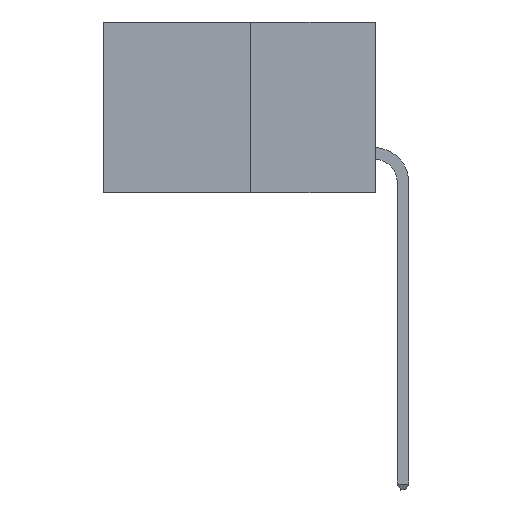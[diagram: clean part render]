
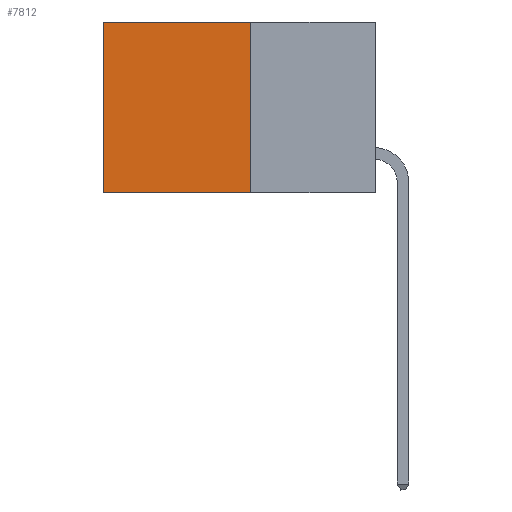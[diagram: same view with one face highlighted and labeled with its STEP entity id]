
A CAD part, left-side view. The second image highlights one B-rep face of the part: STEP entity #7812.
In plain terms, the highlighted planar face has unit normal (-1, 0, 0).
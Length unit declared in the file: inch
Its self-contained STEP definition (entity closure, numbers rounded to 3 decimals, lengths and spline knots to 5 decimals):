
#153 = VERTEX_POINT ( 'NONE', #9840 ) ;
#2208 = VECTOR ( 'NONE', #5039, 39.37008 ) ;
#2853 = EDGE_CURVE ( 'NONE', #7684, #153, #9256, .T. ) ;
#2869 = DIRECTION ( 'NONE',  ( 0., 0., -1. ) ) ;
#3282 = VECTOR ( 'NONE', #2869, 39.37008 ) ;
#3379 = CARTESIAN_POINT ( 'NONE',  ( 0.277, 0.27, -0.37 ) ) ;
#3427 = DIRECTION ( 'NONE',  ( 0., 0., -1. ) ) ;
#3918 = ORIENTED_EDGE ( 'NONE', *, *, #2853, .F. ) ;
#4128 = EDGE_LOOP ( 'NONE', ( #9489, #12944, #3918, #8191 ) ) ;
#5039 = DIRECTION ( 'NONE',  ( 0., 1., 0. ) ) ;
#5162 = DIRECTION ( 'NONE',  ( 0., 1., 0. ) ) ;
#5212 = CARTESIAN_POINT ( 'NONE',  ( 0.277, 0.59, 0. ) ) ;
#5635 = DIRECTION ( 'NONE',  ( 0., 0., -1. ) ) ;
#6323 = VERTEX_POINT ( 'NONE', #11208 ) ;
#6807 = VERTEX_POINT ( 'NONE', #5212 ) ;
#7485 = CARTESIAN_POINT ( 'NONE',  ( 0.277, 0.27, -0.37 ) ) ;
#7684 = VERTEX_POINT ( 'NONE', #11464 ) ;
#7806 = LINE ( 'NONE', #11505, #13668 ) ;
#7812 = ADVANCED_FACE ( 'NONE', ( #8192 ), #8173, .F. ) ;
#8173 = PLANE ( 'NONE',  #9640 ) ;
#8191 = ORIENTED_EDGE ( 'NONE', *, *, #9675, .T. ) ;
#8192 = FACE_OUTER_BOUND ( 'NONE', #4128, .T. ) ;
#9256 = LINE ( 'NONE', #3379, #3282 ) ;
#9312 = LINE ( 'NONE', #10989, #2208 ) ;
#9366 = CARTESIAN_POINT ( 'NONE',  ( 0.277, 0.27, -0.37 ) ) ;
#9489 = ORIENTED_EDGE ( 'NONE', *, *, #9718, .T. ) ;
#9640 = AXIS2_PLACEMENT_3D ( 'NONE', #9366, #10567, #3427 ) ;
#9675 = EDGE_CURVE ( 'NONE', #7684, #6807, #9312, .T. ) ;
#9718 = EDGE_CURVE ( 'NONE', #6807, #6323, #7806, .T. ) ;
#9840 = CARTESIAN_POINT ( 'NONE',  ( 0.277, 0.27, -0.37 ) ) ;
#10567 = DIRECTION ( 'NONE',  ( 1., 0., 0. ) ) ;
#10989 = CARTESIAN_POINT ( 'NONE',  ( 0.277, 0.27, 0. ) ) ;
#11208 = CARTESIAN_POINT ( 'NONE',  ( 0.277, 0.59, -0.37 ) ) ;
#11464 = CARTESIAN_POINT ( 'NONE',  ( 0.277, 0.27, 0. ) ) ;
#11505 = CARTESIAN_POINT ( 'NONE',  ( 0.277, 0.59, -0.37 ) ) ;
#11617 = EDGE_CURVE ( 'NONE', #153, #6323, #13819, .T. ) ;
#12944 = ORIENTED_EDGE ( 'NONE', *, *, #11617, .F. ) ;
#13455 = VECTOR ( 'NONE', #5162, 39.37008 ) ;
#13668 = VECTOR ( 'NONE', #5635, 39.37008 ) ;
#13819 = LINE ( 'NONE', #7485, #13455 ) ;
